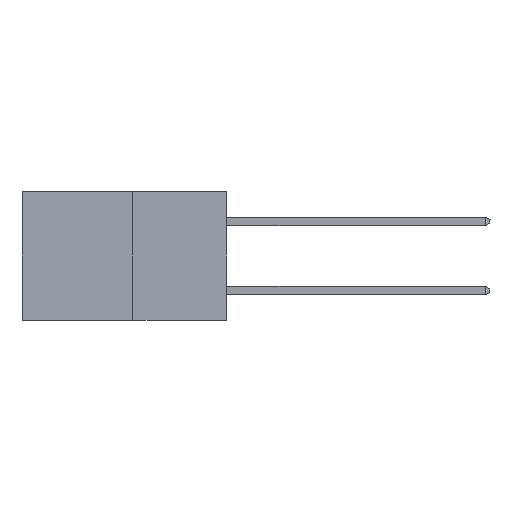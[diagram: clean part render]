
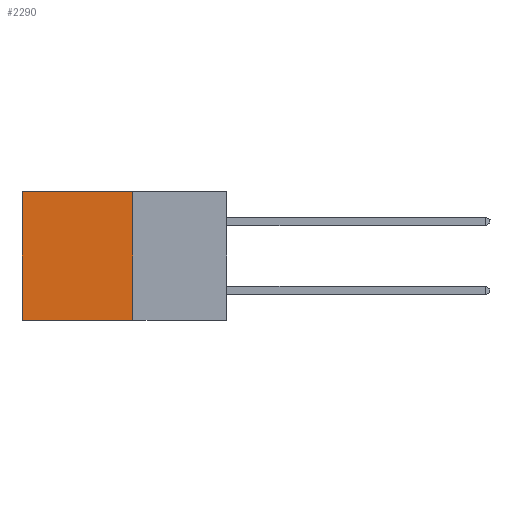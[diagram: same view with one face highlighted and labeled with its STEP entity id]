
A CAD part, left-side view. The second image highlights one B-rep face of the part: STEP entity #2290.
In plain terms, the highlighted planar face has unit normal (-1, 0, 0).
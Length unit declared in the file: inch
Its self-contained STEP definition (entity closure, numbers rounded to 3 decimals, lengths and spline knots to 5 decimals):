
#236 = VERTEX_POINT ( 'NONE', #9030 ) ;
#580 = ORIENTED_EDGE ( 'NONE', *, *, #11650, .T. ) ;
#1144 = ORIENTED_EDGE ( 'NONE', *, *, #1554, .T. ) ;
#1537 = VERTEX_POINT ( 'NONE', #3460 ) ;
#1554 = EDGE_CURVE ( 'NONE', #13524, #236, #14259, .T. ) ;
#1621 = VECTOR ( 'NONE', #8711, 39.37008 ) ;
#1664 = LINE ( 'NONE', #5856, #8541 ) ;
#1992 = LINE ( 'NONE', #8862, #1621 ) ;
#2290 = ADVANCED_FACE ( 'NONE', ( #3704 ), #12083, .F. ) ;
#2442 = CARTESIAN_POINT ( 'NONE',  ( 0.277, 0.27, -0.37 ) ) ;
#3017 = AXIS2_PLACEMENT_3D ( 'NONE', #2442, #6875, #8895 ) ;
#3460 = CARTESIAN_POINT ( 'NONE',  ( 0.277, 0.27, 0. ) ) ;
#3497 = CARTESIAN_POINT ( 'NONE',  ( 0.277, 0.59, 0. ) ) ;
#3650 = EDGE_CURVE ( 'NONE', #7317, #236, #1992, .T. ) ;
#3704 = FACE_OUTER_BOUND ( 'NONE', #5031, .T. ) ;
#4580 = VECTOR ( 'NONE', #5543, 39.37008 ) ;
#5031 = EDGE_LOOP ( 'NONE', ( #1144, #11179, #11940, #580 ) ) ;
#5140 = VECTOR ( 'NONE', #5663, 39.37008 ) ;
#5543 = DIRECTION ( 'NONE',  ( 0., 1., 0. ) ) ;
#5663 = DIRECTION ( 'NONE',  ( 0., 0., -1. ) ) ;
#5856 = CARTESIAN_POINT ( 'NONE',  ( 0.277, 0.27, -0.37 ) ) ;
#5958 = DIRECTION ( 'NONE',  ( 0., 0., -1. ) ) ;
#6875 = DIRECTION ( 'NONE',  ( 1., 0., 0. ) ) ;
#7317 = VERTEX_POINT ( 'NONE', #11880 ) ;
#7439 = LINE ( 'NONE', #12710, #4580 ) ;
#8541 = VECTOR ( 'NONE', #5958, 39.37008 ) ;
#8699 = EDGE_CURVE ( 'NONE', #1537, #7317, #1664, .T. ) ;
#8711 = DIRECTION ( 'NONE',  ( 0., 1., 0. ) ) ;
#8862 = CARTESIAN_POINT ( 'NONE',  ( 0.277, 0.27, -0.37 ) ) ;
#8895 = DIRECTION ( 'NONE',  ( 0., 0., -1. ) ) ;
#9030 = CARTESIAN_POINT ( 'NONE',  ( 0.277, 0.59, -0.37 ) ) ;
#11179 = ORIENTED_EDGE ( 'NONE', *, *, #3650, .F. ) ;
#11413 = CARTESIAN_POINT ( 'NONE',  ( 0.277, 0.59, -0.37 ) ) ;
#11650 = EDGE_CURVE ( 'NONE', #1537, #13524, #7439, .T. ) ;
#11880 = CARTESIAN_POINT ( 'NONE',  ( 0.277, 0.27, -0.37 ) ) ;
#11940 = ORIENTED_EDGE ( 'NONE', *, *, #8699, .F. ) ;
#12083 = PLANE ( 'NONE',  #3017 ) ;
#12710 = CARTESIAN_POINT ( 'NONE',  ( 0.277, 0.27, 0. ) ) ;
#13524 = VERTEX_POINT ( 'NONE', #3497 ) ;
#14259 = LINE ( 'NONE', #11413, #5140 ) ;
